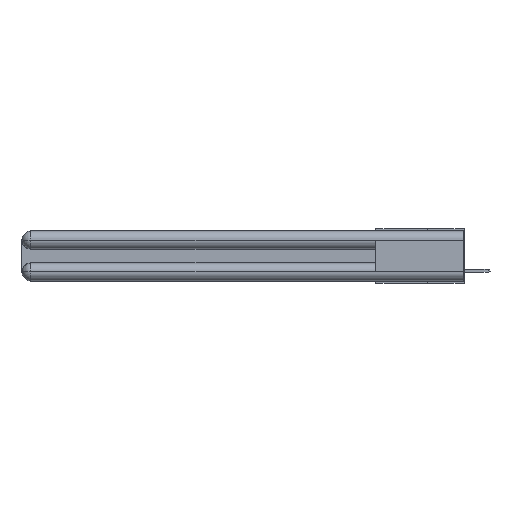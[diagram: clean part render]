
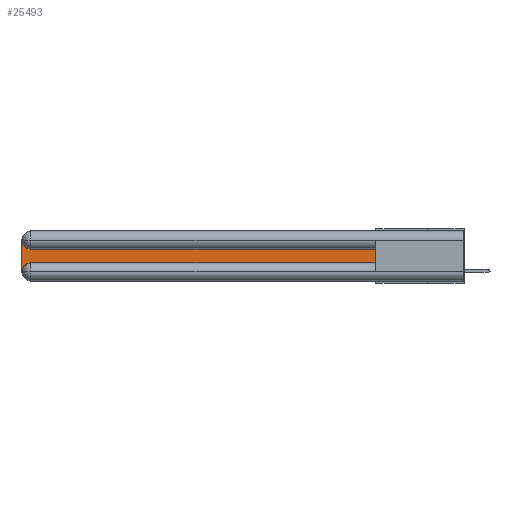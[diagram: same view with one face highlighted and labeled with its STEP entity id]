
A CAD part, left-side view. The second image highlights one B-rep face of the part: STEP entity #25493.
In plain terms, the highlighted planar face has unit normal (-1, 0, 0).
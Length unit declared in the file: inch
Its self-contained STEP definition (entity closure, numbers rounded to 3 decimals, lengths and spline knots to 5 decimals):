
#922 = FACE_OUTER_BOUND ( 'NONE', #19094, .T. ) ;
#2700 = EDGE_CURVE ( 'NONE', #10490, #17550, #27138, .T. ) ;
#3213 = ORIENTED_EDGE ( 'NONE', *, *, #2700, .T. ) ;
#4346 = VECTOR ( 'NONE', #22207, 39.37008 ) ;
#4365 = ORIENTED_EDGE ( 'NONE', *, *, #11420, .T. ) ;
#4696 = LINE ( 'NONE', #5377, #4346 ) ;
#5377 = CARTESIAN_POINT ( 'NONE',  ( 0.075, 3., -0.2175 ) ) ;
#5479 = DIRECTION ( 'NONE',  ( 0., -1., 0. ) ) ;
#5848 = DIRECTION ( 'NONE',  ( 0., 0., -1. ) ) ;
#6157 = CARTESIAN_POINT ( 'NONE',  ( 0.075, 3., -0.1225 ) ) ;
#6168 = CARTESIAN_POINT ( 'NONE',  ( 0.075, 0.6, -0.2175 ) ) ;
#6235 = EDGE_CURVE ( 'NONE', #28869, #19538, #26496, .T. ) ;
#7731 = LINE ( 'NONE', #8072, #24474 ) ;
#8072 = CARTESIAN_POINT ( 'NONE',  ( 0.075, 0.6, -0.2175 ) ) ;
#8959 = DIRECTION ( 'NONE',  ( 0., 0., -1. ) ) ;
#10395 = AXIS2_PLACEMENT_3D ( 'NONE', #20833, #23222, #8959 ) ;
#10490 = VERTEX_POINT ( 'NONE', #18091 ) ;
#10801 = EDGE_CURVE ( 'NONE', #28065, #28869, #4696, .T. ) ;
#11265 = ORIENTED_EDGE ( 'NONE', *, *, #6235, .T. ) ;
#11420 = EDGE_CURVE ( 'NONE', #17550, #18089, #15635, .T. ) ;
#11570 = VECTOR ( 'NONE', #29970, 39.37008 ) ;
#12296 = DIRECTION ( 'NONE',  ( 0., 0., -1. ) ) ;
#13121 = PLANE ( 'NONE',  #25741 ) ;
#14209 = ORIENTED_EDGE ( 'NONE', *, *, #24237, .T. ) ;
#14677 = DIRECTION ( 'NONE',  ( 1., 0., 0. ) ) ;
#15635 = LINE ( 'NONE', #15920, #11570 ) ;
#15920 = CARTESIAN_POINT ( 'NONE',  ( 0.075, 0.6, -0.1225 ) ) ;
#16090 = ORIENTED_EDGE ( 'NONE', *, *, #10801, .T. ) ;
#17550 = VERTEX_POINT ( 'NONE', #24695 ) ;
#18089 = VERTEX_POINT ( 'NONE', #24234 ) ;
#18091 = CARTESIAN_POINT ( 'NONE',  ( 0.075, 0.6, -0.2175 ) ) ;
#18235 = VECTOR ( 'NONE', #25420, 39.37008 ) ;
#19094 = EDGE_LOOP ( 'NONE', ( #4365, #21462, #16090, #11265, #14209, #3213 ) ) ;
#19538 = VERTEX_POINT ( 'NONE', #30030 ) ;
#19984 = DIRECTION ( 'NONE',  ( 1., 0., 0. ) ) ;
#20833 = CARTESIAN_POINT ( 'NONE',  ( 0.075, 2.94, -0.2775 ) ) ;
#21462 = ORIENTED_EDGE ( 'NONE', *, *, #25256, .T. ) ;
#21513 = CARTESIAN_POINT ( 'NONE',  ( 0.075, 3., -0.0625 ) ) ;
#21521 = AXIS2_PLACEMENT_3D ( 'NONE', #24055, #14677, #12296 ) ;
#22207 = DIRECTION ( 'NONE',  ( 0., 0., -1. ) ) ;
#22304 = CARTESIAN_POINT ( 'NONE',  ( 0.075, 3., -0.2775 ) ) ;
#23222 = DIRECTION ( 'NONE',  ( 1., 0., 0. ) ) ;
#24055 = CARTESIAN_POINT ( 'NONE',  ( 0.075, 2.94, -0.0625 ) ) ;
#24234 = CARTESIAN_POINT ( 'NONE',  ( 0.075, 2.94, -0.1225 ) ) ;
#24237 = EDGE_CURVE ( 'NONE', #19538, #10490, #7731, .T. ) ;
#24474 = VECTOR ( 'NONE', #5479, 39.37008 ) ;
#24695 = CARTESIAN_POINT ( 'NONE',  ( 0.075, 0.6, -0.1225 ) ) ;
#25256 = EDGE_CURVE ( 'NONE', #18089, #28065, #25937, .T. ) ;
#25420 = DIRECTION ( 'NONE',  ( 0., 0., 1. ) ) ;
#25493 = ADVANCED_FACE ( 'NONE', ( #922 ), #13121, .F. ) ;
#25741 = AXIS2_PLACEMENT_3D ( 'NONE', #6157, #19984, #5848 ) ;
#25937 = CIRCLE ( 'NONE', #21521, 0.06 ) ;
#26496 = CIRCLE ( 'NONE', #10395, 0.06 ) ;
#27138 = LINE ( 'NONE', #6168, #18235 ) ;
#28065 = VERTEX_POINT ( 'NONE', #21513 ) ;
#28869 = VERTEX_POINT ( 'NONE', #22304 ) ;
#29970 = DIRECTION ( 'NONE',  ( 0., 1., 0. ) ) ;
#30030 = CARTESIAN_POINT ( 'NONE',  ( 0.075, 2.94, -0.2175 ) ) ;
